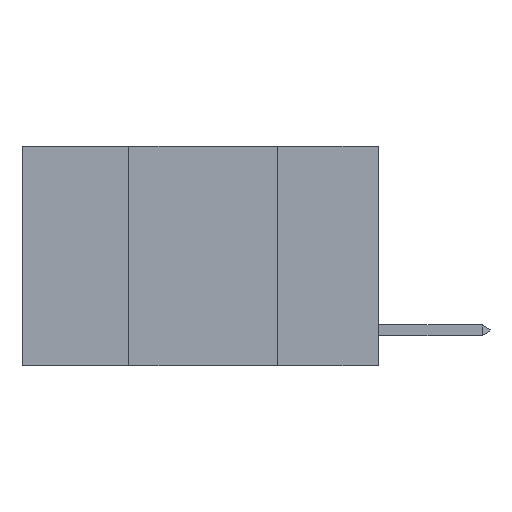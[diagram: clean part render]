
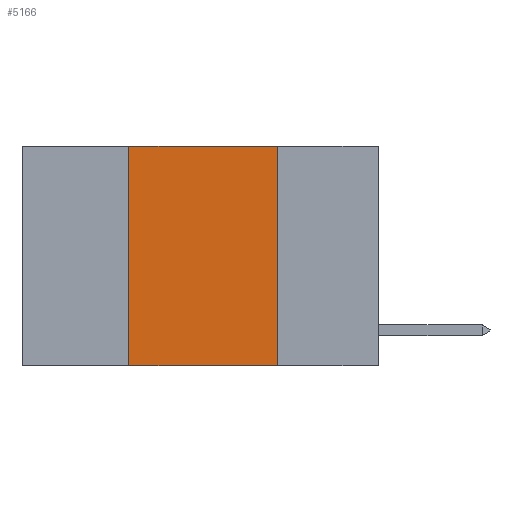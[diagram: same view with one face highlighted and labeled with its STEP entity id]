
A CAD part, left-side view. The second image highlights one B-rep face of the part: STEP entity #5166.
In plain terms, the highlighted planar face has unit normal (-1, 0, 0).
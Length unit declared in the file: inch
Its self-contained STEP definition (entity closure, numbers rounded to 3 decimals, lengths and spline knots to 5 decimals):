
#663 = CARTESIAN_POINT ( 'NONE',  ( 0., 0.17, 0. ) ) ;
#866 = VERTEX_POINT ( 'NONE', #2813 ) ;
#1539 = ORIENTED_EDGE ( 'NONE', *, *, #10751, .F. ) ;
#1598 = AXIS2_PLACEMENT_3D ( 'NONE', #4596, #4717, #8399 ) ;
#1842 = PLANE ( 'NONE',  #1598 ) ;
#2813 = CARTESIAN_POINT ( 'NONE',  ( 0., 0.17, -0.37 ) ) ;
#3414 = DIRECTION ( 'NONE',  ( 0., 0., -1. ) ) ;
#3841 = VERTEX_POINT ( 'NONE', #9166 ) ;
#4182 = CARTESIAN_POINT ( 'NONE',  ( 0., 0.6, 0. ) ) ;
#4596 = CARTESIAN_POINT ( 'NONE',  ( 0., 0.6, 0. ) ) ;
#4717 = DIRECTION ( 'NONE',  ( 1., 0., 0. ) ) ;
#4796 = VERTEX_POINT ( 'NONE', #8493 ) ;
#5164 = LINE ( 'NONE', #4182, #6419 ) ;
#5166 = ADVANCED_FACE ( 'NONE', ( #5536 ), #1842, .F. ) ;
#5455 = LINE ( 'NONE', #7450, #6408 ) ;
#5536 = FACE_OUTER_BOUND ( 'NONE', #9367, .T. ) ;
#5745 = ORIENTED_EDGE ( 'NONE', *, *, #11019, .T. ) ;
#6408 = VECTOR ( 'NONE', #9223, 39.37008 ) ;
#6419 = VECTOR ( 'NONE', #7976, 39.37008 ) ;
#6795 = LINE ( 'NONE', #10582, #11090 ) ;
#7450 = CARTESIAN_POINT ( 'NONE',  ( 0., 0.42, 0. ) ) ;
#7976 = DIRECTION ( 'NONE',  ( 0., -1., 0. ) ) ;
#8399 = DIRECTION ( 'NONE',  ( 0., 0., -1. ) ) ;
#8493 = CARTESIAN_POINT ( 'NONE',  ( 0., 0.17, 0. ) ) ;
#8608 = VECTOR ( 'NONE', #3414, 39.37008 ) ;
#9137 = LINE ( 'NONE', #663, #8608 ) ;
#9166 = CARTESIAN_POINT ( 'NONE',  ( 0., 0.42, -0.37 ) ) ;
#9223 = DIRECTION ( 'NONE',  ( 0., 0., 1. ) ) ;
#9243 = ORIENTED_EDGE ( 'NONE', *, *, #9563, .F. ) ;
#9367 = EDGE_LOOP ( 'NONE', ( #1539, #11498, #9243, #5745 ) ) ;
#9563 = EDGE_CURVE ( 'NONE', #3841, #12118, #5455, .T. ) ;
#10030 = EDGE_CURVE ( 'NONE', #12118, #4796, #5164, .T. ) ;
#10408 = CARTESIAN_POINT ( 'NONE',  ( 0., 0.42, 0. ) ) ;
#10582 = CARTESIAN_POINT ( 'NONE',  ( 0., 0.6, -0.37 ) ) ;
#10751 = EDGE_CURVE ( 'NONE', #4796, #866, #9137, .T. ) ;
#11019 = EDGE_CURVE ( 'NONE', #3841, #866, #6795, .T. ) ;
#11090 = VECTOR ( 'NONE', #11461, 39.37008 ) ;
#11461 = DIRECTION ( 'NONE',  ( 0., -1., 0. ) ) ;
#11498 = ORIENTED_EDGE ( 'NONE', *, *, #10030, .F. ) ;
#12118 = VERTEX_POINT ( 'NONE', #10408 ) ;
